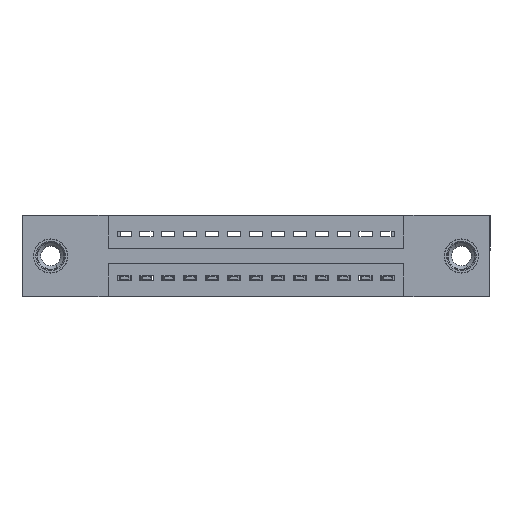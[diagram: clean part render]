
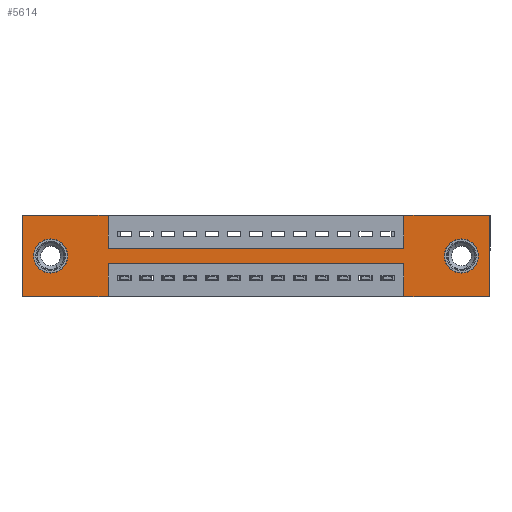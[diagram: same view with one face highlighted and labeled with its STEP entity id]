
A CAD part, front view. The second image highlights one B-rep face of the part: STEP entity #5614.
In plain terms, the highlighted planar face has unit normal (0, -1, 0).
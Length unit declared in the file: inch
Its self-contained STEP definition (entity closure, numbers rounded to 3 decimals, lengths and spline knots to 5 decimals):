
#391 = CARTESIAN_POINT ( 'NONE',  ( 0.3925, 0., -0.22 ) ) ;
#472 = EDGE_CURVE ( 'NONE', #14077, #6717, #14999, .T. ) ;
#481 = CARTESIAN_POINT ( 'NONE',  ( 0., 0., 0. ) ) ;
#486 = LINE ( 'NONE', #9300, #16338 ) ;
#939 = EDGE_LOOP ( 'NONE', ( #3476, #2793 ) ) ;
#1139 = CARTESIAN_POINT ( 'NONE',  ( 0.3925, 0., -0.15 ) ) ;
#1177 = DIRECTION ( 'NONE',  ( 0., 0., 1. ) ) ;
#1319 = VERTEX_POINT ( 'NONE', #8373 ) ;
#1335 = VERTEX_POINT ( 'NONE', #15428 ) ;
#1363 = VERTEX_POINT ( 'NONE', #1510 ) ;
#1510 = CARTESIAN_POINT ( 'NONE',  ( 2.005, 0., -0.263 ) ) ;
#1608 = VERTEX_POINT ( 'NONE', #14888 ) ;
#1700 = PLANE ( 'NONE',  #8428 ) ;
#1772 = CARTESIAN_POINT ( 'NONE',  ( 0., 0., -0.37 ) ) ;
#1830 = CARTESIAN_POINT ( 'NONE',  ( 2.135, 0., 0. ) ) ;
#1860 = CIRCLE ( 'NONE', #17208, 0.078 ) ;
#2125 = ORIENTED_EDGE ( 'NONE', *, *, #4052, .F. ) ;
#2518 = LINE ( 'NONE', #1772, #6908 ) ;
#2572 = DIRECTION ( 'NONE',  ( 0., 0., -1. ) ) ;
#2638 = DIRECTION ( 'NONE',  ( 1., 0., 0. ) ) ;
#2750 = DIRECTION ( 'NONE',  ( 0., 0., -1. ) ) ;
#2793 = ORIENTED_EDGE ( 'NONE', *, *, #472, .T. ) ;
#2986 = ORIENTED_EDGE ( 'NONE', *, *, #14749, .F. ) ;
#3023 = LINE ( 'NONE', #17306, #13775 ) ;
#3064 = EDGE_CURVE ( 'NONE', #1319, #17480, #10809, .T. ) ;
#3094 = DIRECTION ( 'NONE',  ( -1., 0., 0. ) ) ;
#3199 = VERTEX_POINT ( 'NONE', #1830 ) ;
#3309 = CARTESIAN_POINT ( 'NONE',  ( 1.7425, 0., 0. ) ) ;
#3451 = DIRECTION ( 'NONE',  ( 0., 1., 0. ) ) ;
#3462 = EDGE_CURVE ( 'NONE', #4813, #9577, #15361, .T. ) ;
#3469 = DIRECTION ( 'NONE',  ( 1., 0., 0. ) ) ;
#3476 = ORIENTED_EDGE ( 'NONE', *, *, #6032, .T. ) ;
#3505 = CARTESIAN_POINT ( 'NONE',  ( 0.13, 0., -0.185 ) ) ;
#3782 = CARTESIAN_POINT ( 'NONE',  ( 0.13, 0., -0.107 ) ) ;
#4042 = EDGE_CURVE ( 'NONE', #9577, #1319, #10116, .T. ) ;
#4052 = EDGE_CURVE ( 'NONE', #4287, #9195, #5226, .T. ) ;
#4178 = EDGE_CURVE ( 'NONE', #1608, #12239, #3023, .T. ) ;
#4266 = DIRECTION ( 'NONE',  ( 0., 1., 0. ) ) ;
#4287 = VERTEX_POINT ( 'NONE', #6156 ) ;
#4649 = ORIENTED_EDGE ( 'NONE', *, *, #9673, .T. ) ;
#4764 = EDGE_CURVE ( 'NONE', #1363, #1335, #14191, .T. ) ;
#4813 = VERTEX_POINT ( 'NONE', #14260 ) ;
#4892 = VECTOR ( 'NONE', #2638, 39.37008 ) ;
#4952 = FACE_BOUND ( 'NONE', #9359, .T. ) ;
#5079 = DIRECTION ( 'NONE',  ( 0., 0., 1. ) ) ;
#5226 = LINE ( 'NONE', #10276, #11839 ) ;
#5438 = EDGE_CURVE ( 'NONE', #17218, #4813, #2518, .T. ) ;
#5501 = LINE ( 'NONE', #481, #12573 ) ;
#5614 = ADVANCED_FACE ( 'NONE', ( #4952, #7836, #11788 ), #1700, .T. ) ;
#6010 = DIRECTION ( 'NONE',  ( 0., 0., -1. ) ) ;
#6026 = ORIENTED_EDGE ( 'NONE', *, *, #4042, .F. ) ;
#6032 = EDGE_CURVE ( 'NONE', #6717, #14077, #16816, .T. ) ;
#6156 = CARTESIAN_POINT ( 'NONE',  ( 2.135, 0., -0.37 ) ) ;
#6260 = DIRECTION ( 'NONE',  ( 0., 0., 1. ) ) ;
#6717 = VERTEX_POINT ( 'NONE', #3782 ) ;
#6908 = VECTOR ( 'NONE', #15926, 39.37008 ) ;
#6949 = DIRECTION ( 'NONE',  ( 1., 0., 0. ) ) ;
#7065 = CARTESIAN_POINT ( 'NONE',  ( 0.13, 0., -0.263 ) ) ;
#7093 = ORIENTED_EDGE ( 'NONE', *, *, #5438, .F. ) ;
#7098 = CARTESIAN_POINT ( 'NONE',  ( 0., 0., 0. ) ) ;
#7300 = LINE ( 'NONE', #11099, #4892 ) ;
#7414 = DIRECTION ( 'NONE',  ( -1., 0., 0. ) ) ;
#7457 = CARTESIAN_POINT ( 'NONE',  ( 0., 0., -0.37 ) ) ;
#7836 = FACE_BOUND ( 'NONE', #939, .T. ) ;
#7882 = ORIENTED_EDGE ( 'NONE', *, *, #4764, .T. ) ;
#7906 = ORIENTED_EDGE ( 'NONE', *, *, #3462, .F. ) ;
#8297 = EDGE_CURVE ( 'NONE', #9044, #3199, #5501, .T. ) ;
#8305 = VECTOR ( 'NONE', #6949, 39.37008 ) ;
#8373 = CARTESIAN_POINT ( 'NONE',  ( 0.3925, 0., 0. ) ) ;
#8379 = ORIENTED_EDGE ( 'NONE', *, *, #17142, .F. ) ;
#8421 = CARTESIAN_POINT ( 'NONE',  ( 0.3925, 0., 0. ) ) ;
#8428 = AXIS2_PLACEMENT_3D ( 'NONE', #7457, #10191, #6010 ) ;
#8593 = EDGE_CURVE ( 'NONE', #3199, #4287, #18057, .T. ) ;
#8632 = CARTESIAN_POINT ( 'NONE',  ( 0., 0., 0. ) ) ;
#9044 = VERTEX_POINT ( 'NONE', #3309 ) ;
#9195 = VERTEX_POINT ( 'NONE', #11727 ) ;
#9300 = CARTESIAN_POINT ( 'NONE',  ( 1.7425, 0., 0. ) ) ;
#9359 = EDGE_LOOP ( 'NONE', ( #4649, #7882 ) ) ;
#9555 = ORIENTED_EDGE ( 'NONE', *, *, #13633, .F. ) ;
#9577 = VERTEX_POINT ( 'NONE', #9721 ) ;
#9673 = EDGE_CURVE ( 'NONE', #1335, #1363, #1860, .T. ) ;
#9721 = CARTESIAN_POINT ( 'NONE',  ( 0., 0., 0. ) ) ;
#10116 = LINE ( 'NONE', #8632, #8305 ) ;
#10144 = ORIENTED_EDGE ( 'NONE', *, *, #12053, .F. ) ;
#10178 = AXIS2_PLACEMENT_3D ( 'NONE', #3505, #3451, #6260 ) ;
#10191 = DIRECTION ( 'NONE',  ( 0., -1., 0. ) ) ;
#10276 = CARTESIAN_POINT ( 'NONE',  ( 0., 0., -0.37 ) ) ;
#10505 = CARTESIAN_POINT ( 'NONE',  ( 2.005, 0., -0.185 ) ) ;
#10809 = LINE ( 'NONE', #8421, #14946 ) ;
#10929 = DIRECTION ( 'NONE',  ( 0., 0., 1. ) ) ;
#11087 = CARTESIAN_POINT ( 'NONE',  ( 1.7425, 0., -0.37 ) ) ;
#11099 = CARTESIAN_POINT ( 'NONE',  ( 0.3925, 0., -0.15 ) ) ;
#11159 = DIRECTION ( 'NONE',  ( 0., 0., -1. ) ) ;
#11231 = VECTOR ( 'NONE', #10929, 39.37008 ) ;
#11727 = CARTESIAN_POINT ( 'NONE',  ( 1.7425, 0., -0.37 ) ) ;
#11786 = LINE ( 'NONE', #18169, #13099 ) ;
#11788 = FACE_OUTER_BOUND ( 'NONE', #18201, .T. ) ;
#11839 = VECTOR ( 'NONE', #7414, 39.37008 ) ;
#12053 = EDGE_CURVE ( 'NONE', #14155, #9044, #486, .T. ) ;
#12239 = VERTEX_POINT ( 'NONE', #391 ) ;
#12408 = ORIENTED_EDGE ( 'NONE', *, *, #8297, .F. ) ;
#12442 = CARTESIAN_POINT ( 'NONE',  ( 2.005, 0., -0.185 ) ) ;
#12573 = VECTOR ( 'NONE', #3469, 39.37008 ) ;
#12901 = AXIS2_PLACEMENT_3D ( 'NONE', #12442, #4266, #11159 ) ;
#13099 = VECTOR ( 'NONE', #2572, 39.37008 ) ;
#13108 = ORIENTED_EDGE ( 'NONE', *, *, #3064, .F. ) ;
#13303 = CARTESIAN_POINT ( 'NONE',  ( 0.3925, 0., -0.37 ) ) ;
#13606 = LINE ( 'NONE', #11087, #11231 ) ;
#13633 = EDGE_CURVE ( 'NONE', #17480, #14155, #7300, .T. ) ;
#13655 = ORIENTED_EDGE ( 'NONE', *, *, #4178, .F. ) ;
#13687 = DIRECTION ( 'NONE',  ( 0., 1., 0. ) ) ;
#13775 = VECTOR ( 'NONE', #3094, 39.37008 ) ;
#14020 = DIRECTION ( 'NONE',  ( 0., 0., 1. ) ) ;
#14077 = VERTEX_POINT ( 'NONE', #7065 ) ;
#14155 = VERTEX_POINT ( 'NONE', #14211 ) ;
#14191 = CIRCLE ( 'NONE', #12901, 0.078 ) ;
#14211 = CARTESIAN_POINT ( 'NONE',  ( 1.7425, 0., -0.15 ) ) ;
#14244 = DIRECTION ( 'NONE',  ( 0., 0., -1. ) ) ;
#14260 = CARTESIAN_POINT ( 'NONE',  ( 0., 0., -0.37 ) ) ;
#14681 = DIRECTION ( 'NONE',  ( 0., 0., -1. ) ) ;
#14749 = EDGE_CURVE ( 'NONE', #9195, #1608, #13606, .T. ) ;
#14888 = CARTESIAN_POINT ( 'NONE',  ( 1.7425, 0., -0.22 ) ) ;
#14946 = VECTOR ( 'NONE', #14244, 39.37008 ) ;
#14999 = CIRCLE ( 'NONE', #10178, 0.078 ) ;
#15195 = VECTOR ( 'NONE', #2750, 39.37008 ) ;
#15361 = LINE ( 'NONE', #7098, #17789 ) ;
#15428 = CARTESIAN_POINT ( 'NONE',  ( 2.005, 0., -0.107 ) ) ;
#15609 = AXIS2_PLACEMENT_3D ( 'NONE', #17983, #13687, #1177 ) ;
#15840 = DIRECTION ( 'NONE',  ( 0., 1., 0. ) ) ;
#15926 = DIRECTION ( 'NONE',  ( -1., 0., 0. ) ) ;
#16338 = VECTOR ( 'NONE', #5079, 39.37008 ) ;
#16766 = CARTESIAN_POINT ( 'NONE',  ( 2.135, 0., 0. ) ) ;
#16816 = CIRCLE ( 'NONE', #15609, 0.078 ) ;
#17142 = EDGE_CURVE ( 'NONE', #12239, #17218, #11786, .T. ) ;
#17208 = AXIS2_PLACEMENT_3D ( 'NONE', #10505, #15840, #14681 ) ;
#17218 = VERTEX_POINT ( 'NONE', #13303 ) ;
#17267 = ORIENTED_EDGE ( 'NONE', *, *, #8593, .F. ) ;
#17306 = CARTESIAN_POINT ( 'NONE',  ( 0.3925, 0., -0.22 ) ) ;
#17480 = VERTEX_POINT ( 'NONE', #1139 ) ;
#17789 = VECTOR ( 'NONE', #14020, 39.37008 ) ;
#17983 = CARTESIAN_POINT ( 'NONE',  ( 0.13, 0., -0.185 ) ) ;
#18057 = LINE ( 'NONE', #16766, #15195 ) ;
#18169 = CARTESIAN_POINT ( 'NONE',  ( 0.3925, 0., -0.37 ) ) ;
#18201 = EDGE_LOOP ( 'NONE', ( #8379, #13655, #2986, #2125, #17267, #12408, #10144, #9555, #13108, #6026, #7906, #7093 ) ) ;
